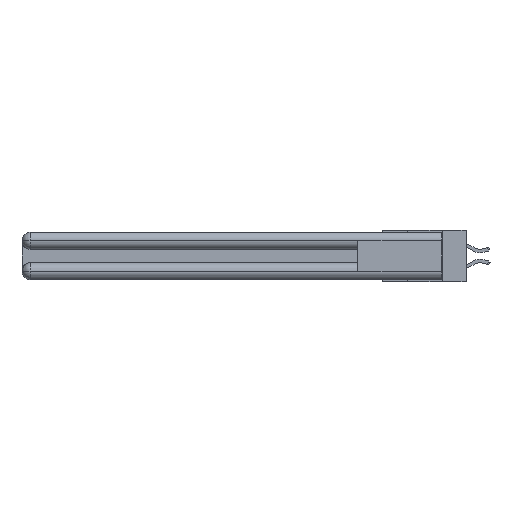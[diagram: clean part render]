
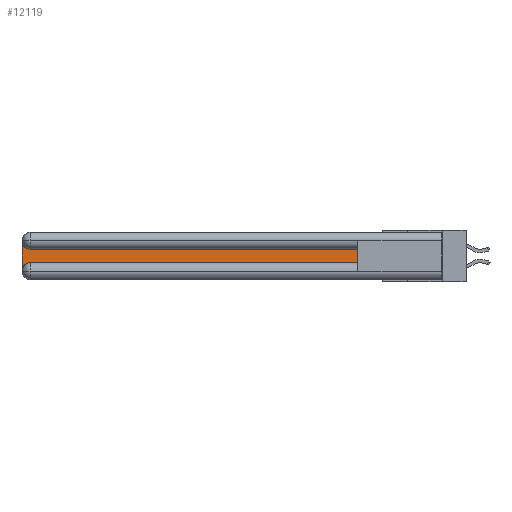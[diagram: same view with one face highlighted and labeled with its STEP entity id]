
A CAD part, left-side view. The second image highlights one B-rep face of the part: STEP entity #12119.
In plain terms, the highlighted planar face has unit normal (-1, 0, 0).
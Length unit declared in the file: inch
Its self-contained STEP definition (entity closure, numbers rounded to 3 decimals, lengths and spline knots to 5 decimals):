
#1119 = CARTESIAN_POINT ( 'NONE',  ( 0.075, 2.94, -0.0625 ) ) ;
#1228 = DIRECTION ( 'NONE',  ( 1., 0., 0. ) ) ;
#1801 = DIRECTION ( 'NONE',  ( 0., -1., 0. ) ) ;
#2607 = AXIS2_PLACEMENT_3D ( 'NONE', #1119, #1228, #3638 ) ;
#3346 = EDGE_CURVE ( 'NONE', #18987, #30223, #9982, .T. ) ;
#3638 = DIRECTION ( 'NONE',  ( 0., 0., -1. ) ) ;
#4442 = VERTEX_POINT ( 'NONE', #9390 ) ;
#5031 = CARTESIAN_POINT ( 'NONE',  ( 0.075, 3., -0.1225 ) ) ;
#5157 = ORIENTED_EDGE ( 'NONE', *, *, #3346, .T. ) ;
#5954 = LINE ( 'NONE', #30409, #15714 ) ;
#6453 = FACE_OUTER_BOUND ( 'NONE', #9793, .T. ) ;
#6663 = CARTESIAN_POINT ( 'NONE',  ( 0.075, 0.6, -0.1225 ) ) ;
#7294 = DIRECTION ( 'NONE',  ( 1., 0., 0. ) ) ;
#8541 = AXIS2_PLACEMENT_3D ( 'NONE', #22381, #7294, #17077 ) ;
#8800 = CARTESIAN_POINT ( 'NONE',  ( 0.075, 2.94, -0.1225 ) ) ;
#9235 = ORIENTED_EDGE ( 'NONE', *, *, #16713, .T. ) ;
#9239 = VECTOR ( 'NONE', #16982, 39.37008 ) ;
#9390 = CARTESIAN_POINT ( 'NONE',  ( 0.075, 0.6, -0.1225 ) ) ;
#9793 = EDGE_LOOP ( 'NONE', ( #9877, #9235, #31609, #5157, #23628, #11542 ) ) ;
#9877 = ORIENTED_EDGE ( 'NONE', *, *, #11381, .T. ) ;
#9982 = CIRCLE ( 'NONE', #8541, 0.06 ) ;
#10263 = AXIS2_PLACEMENT_3D ( 'NONE', #5031, #15265, #25396 ) ;
#11296 = CIRCLE ( 'NONE', #2607, 0.06 ) ;
#11381 = EDGE_CURVE ( 'NONE', #4442, #19889, #15845, .T. ) ;
#11542 = ORIENTED_EDGE ( 'NONE', *, *, #20101, .T. ) ;
#12119 = ADVANCED_FACE ( 'NONE', ( #6453 ), #22749, .F. ) ;
#12186 = VECTOR ( 'NONE', #25921, 39.37008 ) ;
#15265 = DIRECTION ( 'NONE',  ( 1., 0., 0. ) ) ;
#15714 = VECTOR ( 'NONE', #18140, 39.37008 ) ;
#15845 = LINE ( 'NONE', #6663, #9239 ) ;
#16384 = LINE ( 'NONE', #31963, #28164 ) ;
#16713 = EDGE_CURVE ( 'NONE', #19889, #28022, #11296, .T. ) ;
#16982 = DIRECTION ( 'NONE',  ( 0., 1., 0. ) ) ;
#17077 = DIRECTION ( 'NONE',  ( 0., 0., -1. ) ) ;
#18140 = DIRECTION ( 'NONE',  ( 0., 0., 1. ) ) ;
#18987 = VERTEX_POINT ( 'NONE', #22365 ) ;
#19355 = VERTEX_POINT ( 'NONE', #21371 ) ;
#19889 = VERTEX_POINT ( 'NONE', #8800 ) ;
#20101 = EDGE_CURVE ( 'NONE', #19355, #4442, #5954, .T. ) ;
#20547 = EDGE_CURVE ( 'NONE', #28022, #18987, #31744, .T. ) ;
#21371 = CARTESIAN_POINT ( 'NONE',  ( 0.075, 0.6, -0.2175 ) ) ;
#22365 = CARTESIAN_POINT ( 'NONE',  ( 0.075, 3., -0.2775 ) ) ;
#22381 = CARTESIAN_POINT ( 'NONE',  ( 0.075, 2.94, -0.2775 ) ) ;
#22749 = PLANE ( 'NONE',  #10263 ) ;
#23628 = ORIENTED_EDGE ( 'NONE', *, *, #26460, .T. ) ;
#25396 = DIRECTION ( 'NONE',  ( 0., 0., -1. ) ) ;
#25921 = DIRECTION ( 'NONE',  ( 0., 0., -1. ) ) ;
#26460 = EDGE_CURVE ( 'NONE', #30223, #19355, #16384, .T. ) ;
#28022 = VERTEX_POINT ( 'NONE', #30410 ) ;
#28164 = VECTOR ( 'NONE', #1801, 39.37008 ) ;
#28183 = CARTESIAN_POINT ( 'NONE',  ( 0.075, 3., -0.2175 ) ) ;
#30223 = VERTEX_POINT ( 'NONE', #31519 ) ;
#30409 = CARTESIAN_POINT ( 'NONE',  ( 0.075, 0.6, -0.2175 ) ) ;
#30410 = CARTESIAN_POINT ( 'NONE',  ( 0.075, 3., -0.0625 ) ) ;
#31519 = CARTESIAN_POINT ( 'NONE',  ( 0.075, 2.94, -0.2175 ) ) ;
#31609 = ORIENTED_EDGE ( 'NONE', *, *, #20547, .T. ) ;
#31744 = LINE ( 'NONE', #28183, #12186 ) ;
#31963 = CARTESIAN_POINT ( 'NONE',  ( 0.075, 0.6, -0.2175 ) ) ;
